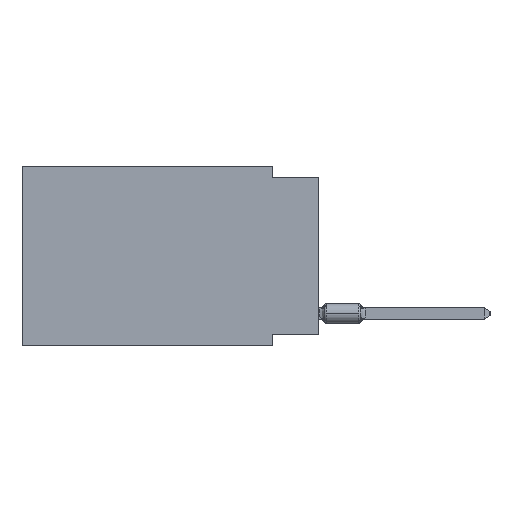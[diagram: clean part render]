
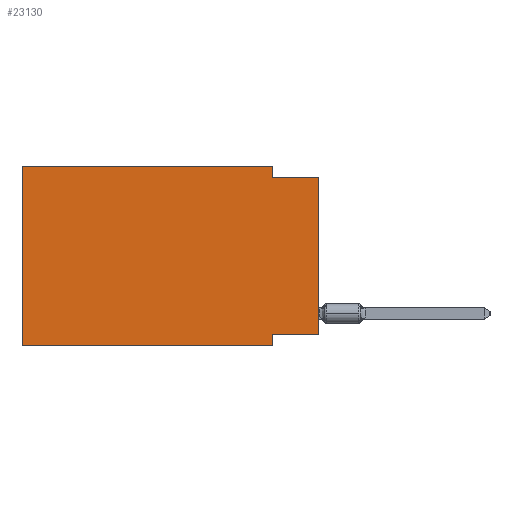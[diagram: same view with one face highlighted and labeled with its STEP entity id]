
A CAD part, left-side view. The second image highlights one B-rep face of the part: STEP entity #23130.
In plain terms, the highlighted planar face has unit normal (-1, 0, 0).
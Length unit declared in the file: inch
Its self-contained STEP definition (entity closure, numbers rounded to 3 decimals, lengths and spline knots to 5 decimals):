
#304 = EDGE_CURVE ( 'NONE', #1531, #17275, #30306, .T. ) ;
#1530 = ORIENTED_EDGE ( 'NONE', *, *, #31559, .F. ) ;
#1531 = VERTEX_POINT ( 'NONE', #7619 ) ;
#1929 = LINE ( 'NONE', #16440, #9404 ) ;
#2217 = VECTOR ( 'NONE', #24572, 39.37008 ) ;
#2369 = DIRECTION ( 'NONE',  ( 0., 1., 0. ) ) ;
#2710 = EDGE_LOOP ( 'NONE', ( #17277, #26671, #8487, #1530, #5439, #12041, #39191, #5735 ) ) ;
#2808 = EDGE_CURVE ( 'NONE', #3985, #10316, #5294, .T. ) ;
#3301 = LINE ( 'NONE', #20703, #9258 ) ;
#3447 = VECTOR ( 'NONE', #8873, 39.37008 ) ;
#3985 = VERTEX_POINT ( 'NONE', #21018 ) ;
#4522 = CARTESIAN_POINT ( 'NONE',  ( 0., 0.645, 0. ) ) ;
#5294 = LINE ( 'NONE', #45244, #17734 ) ;
#5439 = ORIENTED_EDGE ( 'NONE', *, *, #304, .F. ) ;
#5735 = ORIENTED_EDGE ( 'NONE', *, *, #18588, .F. ) ;
#7041 = CARTESIAN_POINT ( 'NONE',  ( 0., 0.645, 0. ) ) ;
#7619 = CARTESIAN_POINT ( 'NONE',  ( 0., 0.645, -0.39 ) ) ;
#8487 = ORIENTED_EDGE ( 'NONE', *, *, #2808, .F. ) ;
#8740 = VERTEX_POINT ( 'NONE', #24015 ) ;
#8873 = DIRECTION ( 'NONE',  ( 0., 0., 1. ) ) ;
#9258 = VECTOR ( 'NONE', #2369, 39.37008 ) ;
#9404 = VECTOR ( 'NONE', #26956, 39.37008 ) ;
#10026 = EDGE_CURVE ( 'NONE', #12367, #40303, #13062, .T. ) ;
#10316 = VERTEX_POINT ( 'NONE', #18970 ) ;
#11100 = DIRECTION ( 'NONE',  ( 0., -1., 0. ) ) ;
#11332 = CARTESIAN_POINT ( 'NONE',  ( 0., 0.645, -0.39 ) ) ;
#12041 = ORIENTED_EDGE ( 'NONE', *, *, #35959, .T. ) ;
#12367 = VERTEX_POINT ( 'NONE', #27213 ) ;
#13062 = LINE ( 'NONE', #19095, #21900 ) ;
#13110 = EDGE_CURVE ( 'NONE', #10316, #29315, #38363, .T. ) ;
#14963 = CARTESIAN_POINT ( 'NONE',  ( 0., 0., -0.025 ) ) ;
#16440 = CARTESIAN_POINT ( 'NONE',  ( 0., 0.645, 0. ) ) ;
#17275 = VERTEX_POINT ( 'NONE', #4522 ) ;
#17277 = ORIENTED_EDGE ( 'NONE', *, *, #33760, .T. ) ;
#17734 = VECTOR ( 'NONE', #41676, 39.37008 ) ;
#18588 = EDGE_CURVE ( 'NONE', #8740, #12367, #3301, .T. ) ;
#18970 = CARTESIAN_POINT ( 'NONE',  ( 0., 0.1, -0.025 ) ) ;
#19095 = CARTESIAN_POINT ( 'NONE',  ( 0., 0.1, -0.39 ) ) ;
#19600 = AXIS2_PLACEMENT_3D ( 'NONE', #7041, #24687, #29191 ) ;
#20703 = CARTESIAN_POINT ( 'NONE',  ( 0., 0., -0.365 ) ) ;
#21018 = CARTESIAN_POINT ( 'NONE',  ( 0., 0.1, 0. ) ) ;
#21900 = VECTOR ( 'NONE', #42065, 39.37008 ) ;
#22930 = DIRECTION ( 'NONE',  ( 0., 0., 1. ) ) ;
#23130 = ADVANCED_FACE ( 'NONE', ( #45825 ), #23741, .F. ) ;
#23741 = PLANE ( 'NONE',  #19600 ) ;
#24015 = CARTESIAN_POINT ( 'NONE',  ( 0., 0., -0.365 ) ) ;
#24572 = DIRECTION ( 'NONE',  ( 0., -1., 0. ) ) ;
#24687 = DIRECTION ( 'NONE',  ( 1., 0., 0. ) ) ;
#26671 = ORIENTED_EDGE ( 'NONE', *, *, #13110, .F. ) ;
#26956 = DIRECTION ( 'NONE',  ( 0., -1., 0. ) ) ;
#27213 = CARTESIAN_POINT ( 'NONE',  ( 0., 0.1, -0.365 ) ) ;
#29191 = DIRECTION ( 'NONE',  ( 0., 0., -1. ) ) ;
#29315 = VERTEX_POINT ( 'NONE', #14963 ) ;
#30306 = LINE ( 'NONE', #33861, #46060 ) ;
#31559 = EDGE_CURVE ( 'NONE', #17275, #3985, #1929, .T. ) ;
#31939 = CARTESIAN_POINT ( 'NONE',  ( 0., 0.1, -0.39 ) ) ;
#33760 = EDGE_CURVE ( 'NONE', #8740, #29315, #44779, .T. ) ;
#33861 = CARTESIAN_POINT ( 'NONE',  ( 0., 0.645, 0. ) ) ;
#33867 = CARTESIAN_POINT ( 'NONE',  ( 0., 0., 0. ) ) ;
#35959 = EDGE_CURVE ( 'NONE', #1531, #40303, #43685, .T. ) ;
#38125 = CARTESIAN_POINT ( 'NONE',  ( 0., 0., -0.025 ) ) ;
#38363 = LINE ( 'NONE', #38125, #2217 ) ;
#39191 = ORIENTED_EDGE ( 'NONE', *, *, #10026, .F. ) ;
#40303 = VERTEX_POINT ( 'NONE', #31939 ) ;
#41676 = DIRECTION ( 'NONE',  ( 0., 0., -1. ) ) ;
#42065 = DIRECTION ( 'NONE',  ( 0., 0., -1. ) ) ;
#43525 = VECTOR ( 'NONE', #11100, 39.37008 ) ;
#43685 = LINE ( 'NONE', #11332, #43525 ) ;
#44779 = LINE ( 'NONE', #33867, #3447 ) ;
#45244 = CARTESIAN_POINT ( 'NONE',  ( 0., 0.1, 0. ) ) ;
#45825 = FACE_OUTER_BOUND ( 'NONE', #2710, .T. ) ;
#46060 = VECTOR ( 'NONE', #22930, 39.37008 ) ;
